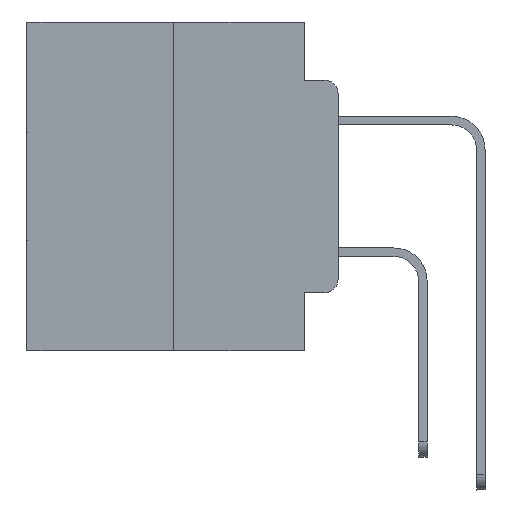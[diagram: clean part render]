
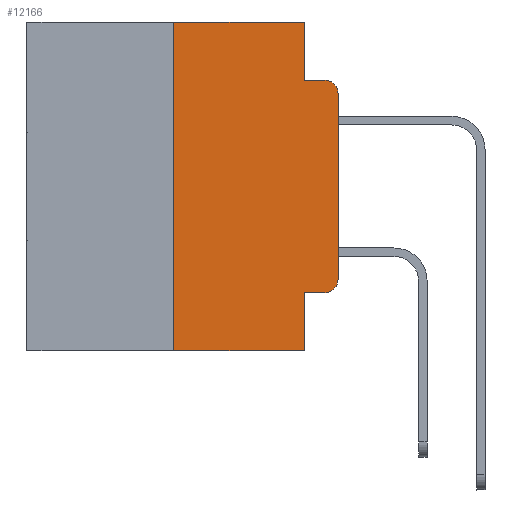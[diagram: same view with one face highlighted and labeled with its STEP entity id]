
A CAD part, left-side view. The second image highlights one B-rep face of the part: STEP entity #12166.
In plain terms, the highlighted planar face has unit normal (-1, 0, 0).
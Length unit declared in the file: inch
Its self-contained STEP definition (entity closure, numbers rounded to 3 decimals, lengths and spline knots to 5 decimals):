
#156 = VERTEX_POINT ( 'NONE', #16644 ) ;
#354 = VECTOR ( 'NONE', #22471, 39.37008 ) ;
#537 = VERTEX_POINT ( 'NONE', #21915 ) ;
#626 = CARTESIAN_POINT ( 'NONE',  ( 0., 0.051, -0.4115 ) ) ;
#1549 = EDGE_CURVE ( 'NONE', #12467, #12633, #4741, .T. ) ;
#2208 = DIRECTION ( 'NONE',  ( -1., 0., 0. ) ) ;
#2406 = CARTESIAN_POINT ( 'NONE',  ( 0., 0.051, -0.0885 ) ) ;
#3075 = EDGE_CURVE ( 'NONE', #23166, #26426, #3791, .T. ) ;
#3241 = CARTESIAN_POINT ( 'NONE',  ( 0., 0., 0. ) ) ;
#3791 = LINE ( 'NONE', #28812, #26655 ) ;
#3878 = CARTESIAN_POINT ( 'NONE',  ( 0., 0., -0.1085 ) ) ;
#4661 = ORIENTED_EDGE ( 'NONE', *, *, #25958, .T. ) ;
#4714 = CARTESIAN_POINT ( 'NONE',  ( 0., 0.051, -0.5 ) ) ;
#4741 = LINE ( 'NONE', #9937, #21857 ) ;
#6138 = EDGE_CURVE ( 'NONE', #26426, #156, #25850, .T. ) ;
#6471 = LINE ( 'NONE', #6905, #354 ) ;
#6753 = CARTESIAN_POINT ( 'NONE',  ( 0., 0.25, -0.5 ) ) ;
#6905 = CARTESIAN_POINT ( 'NONE',  ( 0., 0.051, 0. ) ) ;
#7132 = ORIENTED_EDGE ( 'NONE', *, *, #6138, .F. ) ;
#7303 = VERTEX_POINT ( 'NONE', #3878 ) ;
#7841 = ORIENTED_EDGE ( 'NONE', *, *, #13407, .F. ) ;
#8053 = EDGE_CURVE ( 'NONE', #12467, #26427, #23068, .T. ) ;
#8220 = AXIS2_PLACEMENT_3D ( 'NONE', #22221, #8939, #24392 ) ;
#8939 = DIRECTION ( 'NONE',  ( -1., 0., 0. ) ) ;
#9197 = EDGE_CURVE ( 'NONE', #7303, #156, #18081, .T. ) ;
#9937 = CARTESIAN_POINT ( 'NONE',  ( 0., 0.25, 0. ) ) ;
#10104 = CIRCLE ( 'NONE', #8220, 0.02 ) ;
#10348 = DIRECTION ( 'NONE',  ( 1., 0., 0. ) ) ;
#10688 = EDGE_CURVE ( 'NONE', #12489, #7303, #20357, .T. ) ;
#11030 = VECTOR ( 'NONE', #11963, 39.37008 ) ;
#11963 = DIRECTION ( 'NONE',  ( 0., -1., 0. ) ) ;
#12166 = ADVANCED_FACE ( 'NONE', ( #26342 ), #17007, .F. ) ;
#12467 = VERTEX_POINT ( 'NONE', #6753 ) ;
#12489 = VERTEX_POINT ( 'NONE', #20236 ) ;
#12633 = VERTEX_POINT ( 'NONE', #14003 ) ;
#12968 = LINE ( 'NONE', #27922, #19534 ) ;
#13407 = EDGE_CURVE ( 'NONE', #12633, #23166, #12968, .T. ) ;
#13529 = DIRECTION ( 'NONE',  ( 0., 0., -1. ) ) ;
#13773 = DIRECTION ( 'NONE',  ( 0., -1., 0. ) ) ;
#14003 = CARTESIAN_POINT ( 'NONE',  ( 0., 0.25, 0. ) ) ;
#14241 = DIRECTION ( 'NONE',  ( 0., 0., 1. ) ) ;
#14929 = DIRECTION ( 'NONE',  ( 0., -1., 0. ) ) ;
#15798 = CARTESIAN_POINT ( 'NONE',  ( 0., 0.02, -0.1085 ) ) ;
#16072 = AXIS2_PLACEMENT_3D ( 'NONE', #23591, #10348, #25719 ) ;
#16325 = DIRECTION ( 'NONE',  ( 0., -1., 0. ) ) ;
#16644 = CARTESIAN_POINT ( 'NONE',  ( 0., 0.02, -0.0885 ) ) ;
#17007 = PLANE ( 'NONE',  #16072 ) ;
#17048 = EDGE_LOOP ( 'NONE', ( #23469, #18385, #7132, #19063, #7841, #20401, #26136, #21079, #4661, #23134 ) ) ;
#17290 = VECTOR ( 'NONE', #13773, 39.37008 ) ;
#17507 = VERTEX_POINT ( 'NONE', #26236 ) ;
#18013 = DIRECTION ( 'NONE',  ( 0., 0., -1. ) ) ;
#18081 = CIRCLE ( 'NONE', #28354, 0.02 ) ;
#18385 = ORIENTED_EDGE ( 'NONE', *, *, #9197, .T. ) ;
#18995 = DIRECTION ( 'NONE',  ( 0., 0., 1. ) ) ;
#19063 = ORIENTED_EDGE ( 'NONE', *, *, #3075, .F. ) ;
#19534 = VECTOR ( 'NONE', #14929, 39.37008 ) ;
#20236 = CARTESIAN_POINT ( 'NONE',  ( 0., 0., -0.3915 ) ) ;
#20357 = LINE ( 'NONE', #3241, #24095 ) ;
#20401 = ORIENTED_EDGE ( 'NONE', *, *, #1549, .F. ) ;
#21079 = ORIENTED_EDGE ( 'NONE', *, *, #27400, .F. ) ;
#21857 = VECTOR ( 'NONE', #14241, 39.37008 ) ;
#21915 = CARTESIAN_POINT ( 'NONE',  ( 0., 0.051, -0.4115 ) ) ;
#22221 = CARTESIAN_POINT ( 'NONE',  ( 0., 0.02, -0.3915 ) ) ;
#22471 = DIRECTION ( 'NONE',  ( 0., 0., -1. ) ) ;
#22810 = LINE ( 'NONE', #626, #11030 ) ;
#23068 = LINE ( 'NONE', #26783, #17290 ) ;
#23134 = ORIENTED_EDGE ( 'NONE', *, *, #24528, .T. ) ;
#23166 = VERTEX_POINT ( 'NONE', #27458 ) ;
#23469 = ORIENTED_EDGE ( 'NONE', *, *, #10688, .T. ) ;
#23591 = CARTESIAN_POINT ( 'NONE',  ( 0., 0.473, 0. ) ) ;
#24095 = VECTOR ( 'NONE', #18995, 39.37008 ) ;
#24392 = DIRECTION ( 'NONE',  ( 0., 0., -1. ) ) ;
#24528 = EDGE_CURVE ( 'NONE', #17507, #12489, #10104, .T. ) ;
#25049 = CARTESIAN_POINT ( 'NONE',  ( 0., 0.051, -0.0885 ) ) ;
#25182 = VECTOR ( 'NONE', #16325, 39.37008 ) ;
#25719 = DIRECTION ( 'NONE',  ( 0., 0., -1. ) ) ;
#25850 = LINE ( 'NONE', #25049, #25182 ) ;
#25958 = EDGE_CURVE ( 'NONE', #537, #17507, #22810, .T. ) ;
#26136 = ORIENTED_EDGE ( 'NONE', *, *, #8053, .T. ) ;
#26236 = CARTESIAN_POINT ( 'NONE',  ( 0., 0.02, -0.4115 ) ) ;
#26342 = FACE_OUTER_BOUND ( 'NONE', #17048, .T. ) ;
#26426 = VERTEX_POINT ( 'NONE', #2406 ) ;
#26427 = VERTEX_POINT ( 'NONE', #4714 ) ;
#26655 = VECTOR ( 'NONE', #13529, 39.37008 ) ;
#26783 = CARTESIAN_POINT ( 'NONE',  ( 0., 0.473, -0.5 ) ) ;
#27400 = EDGE_CURVE ( 'NONE', #537, #26427, #6471, .T. ) ;
#27458 = CARTESIAN_POINT ( 'NONE',  ( 0., 0.051, 0. ) ) ;
#27922 = CARTESIAN_POINT ( 'NONE',  ( 0., 0.473, 0. ) ) ;
#28354 = AXIS2_PLACEMENT_3D ( 'NONE', #15798, #2208, #18013 ) ;
#28812 = CARTESIAN_POINT ( 'NONE',  ( 0., 0.051, 0. ) ) ;
